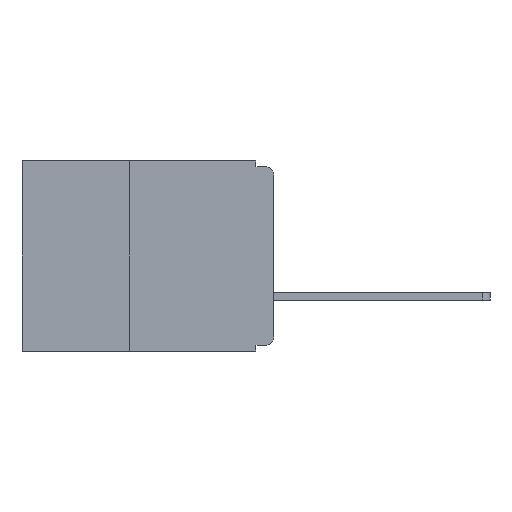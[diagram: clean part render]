
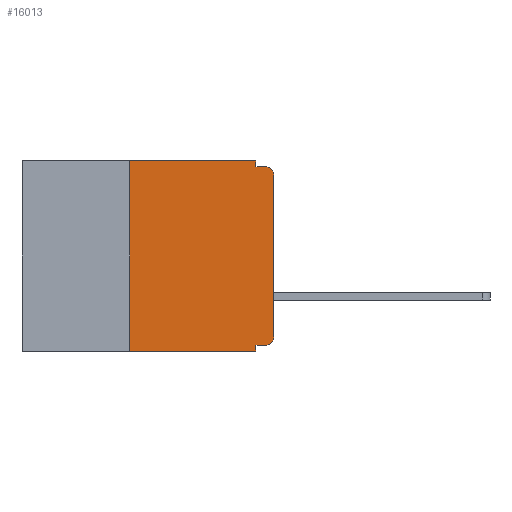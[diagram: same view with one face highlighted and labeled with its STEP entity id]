
A CAD part, left-side view. The second image highlights one B-rep face of the part: STEP entity #16013.
In plain terms, the highlighted planar face has unit normal (-1, 0, 0).
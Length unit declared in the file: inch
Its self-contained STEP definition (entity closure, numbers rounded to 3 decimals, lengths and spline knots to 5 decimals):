
#114 = ORIENTED_EDGE ( 'NONE', *, *, #16668, .T. ) ;
#137 = DIRECTION ( 'NONE',  ( 1., 0., 0. ) ) ;
#272 = CARTESIAN_POINT ( 'NONE',  ( 0., 0., -0.01 ) ) ;
#678 = VERTEX_POINT ( 'NONE', #17223 ) ;
#1757 = CARTESIAN_POINT ( 'NONE',  ( 0., 0.437, -0.33 ) ) ;
#1976 = VECTOR ( 'NONE', #2383, 39.37008 ) ;
#2167 = CARTESIAN_POINT ( 'NONE',  ( 0., 0.25, -0.33 ) ) ;
#2374 = VECTOR ( 'NONE', #10264, 39.37008 ) ;
#2383 = DIRECTION ( 'NONE',  ( 0., -1., 0. ) ) ;
#3712 = VERTEX_POINT ( 'NONE', #26113 ) ;
#4060 = CARTESIAN_POINT ( 'NONE',  ( 0., 0.437, 0. ) ) ;
#4371 = DIRECTION ( 'NONE',  ( 0., 0., -1. ) ) ;
#4772 = ORIENTED_EDGE ( 'NONE', *, *, #26075, .F. ) ;
#5046 = CARTESIAN_POINT ( 'NONE',  ( 0., 0.015, -0.32 ) ) ;
#5273 = EDGE_CURVE ( 'NONE', #24121, #24599, #18374, .T. ) ;
#5412 = CARTESIAN_POINT ( 'NONE',  ( 0., 0.015, -0.01 ) ) ;
#5504 = CARTESIAN_POINT ( 'NONE',  ( 0., 0., -0.305 ) ) ;
#5702 = ORIENTED_EDGE ( 'NONE', *, *, #24195, .T. ) ;
#5765 = ORIENTED_EDGE ( 'NONE', *, *, #13724, .F. ) ;
#5928 = EDGE_CURVE ( 'NONE', #8922, #3712, #12627, .T. ) ;
#6263 = VERTEX_POINT ( 'NONE', #5504 ) ;
#7108 = EDGE_CURVE ( 'NONE', #18911, #24121, #21765, .T. ) ;
#7191 = VERTEX_POINT ( 'NONE', #15669 ) ;
#7644 = VERTEX_POINT ( 'NONE', #23630 ) ;
#7663 = ORIENTED_EDGE ( 'NONE', *, *, #5273, .F. ) ;
#7872 = AXIS2_PLACEMENT_3D ( 'NONE', #8606, #22860, #10690 ) ;
#8042 = DIRECTION ( 'NONE',  ( 0., -1., 0. ) ) ;
#8606 = CARTESIAN_POINT ( 'NONE',  ( 0., 0.015, -0.025 ) ) ;
#8641 = CARTESIAN_POINT ( 'NONE',  ( 0., 0., -0.32 ) ) ;
#8922 = VERTEX_POINT ( 'NONE', #5046 ) ;
#8934 = LINE ( 'NONE', #25769, #25179 ) ;
#9627 = CARTESIAN_POINT ( 'NONE',  ( 0., 0.031, -0.01 ) ) ;
#9970 = CARTESIAN_POINT ( 'NONE',  ( 0., 0.015, -0.305 ) ) ;
#10036 = LINE ( 'NONE', #1757, #20617 ) ;
#10264 = DIRECTION ( 'NONE',  ( 0., 0., -1. ) ) ;
#10690 = DIRECTION ( 'NONE',  ( 0., 0., -1. ) ) ;
#10937 = CIRCLE ( 'NONE', #24810, 0.015 ) ;
#12020 = DIRECTION ( 'NONE',  ( 0., 0., -1. ) ) ;
#12032 = EDGE_CURVE ( 'NONE', #12923, #7644, #10036, .T. ) ;
#12591 = CARTESIAN_POINT ( 'NONE',  ( 0., 0.437, 0. ) ) ;
#12626 = CARTESIAN_POINT ( 'NONE',  ( 0., 0.031, 0. ) ) ;
#12627 = LINE ( 'NONE', #8641, #22792 ) ;
#12755 = LINE ( 'NONE', #16307, #2374 ) ;
#12923 = VERTEX_POINT ( 'NONE', #2167 ) ;
#13618 = DIRECTION ( 'NONE',  ( 0., 0., 1. ) ) ;
#13646 = VECTOR ( 'NONE', #22531, 39.37008 ) ;
#13724 = EDGE_CURVE ( 'NONE', #12923, #678, #8934, .T. ) ;
#14051 = ORIENTED_EDGE ( 'NONE', *, *, #18805, .T. ) ;
#14412 = AXIS2_PLACEMENT_3D ( 'NONE', #12591, #137, #14655 ) ;
#14655 = DIRECTION ( 'NONE',  ( 0., 0., -1. ) ) ;
#15669 = CARTESIAN_POINT ( 'NONE',  ( 0., 0., -0.025 ) ) ;
#16013 = ADVANCED_FACE ( 'NONE', ( #25985 ), #20676, .F. ) ;
#16049 = DIRECTION ( 'NONE',  ( 0., 0., 1. ) ) ;
#16307 = CARTESIAN_POINT ( 'NONE',  ( 0., 0.031, -0.33 ) ) ;
#16668 = EDGE_CURVE ( 'NONE', #7191, #24599, #25005, .T. ) ;
#17105 = LINE ( 'NONE', #26169, #21230 ) ;
#17223 = CARTESIAN_POINT ( 'NONE',  ( 0., 0.25, 0. ) ) ;
#18302 = EDGE_LOOP ( 'NONE', ( #5702, #114, #7663, #21236, #4772, #5765, #26265, #18310, #24473, #14051 ) ) ;
#18310 = ORIENTED_EDGE ( 'NONE', *, *, #22620, .F. ) ;
#18374 = LINE ( 'NONE', #272, #1976 ) ;
#18805 = EDGE_CURVE ( 'NONE', #8922, #6263, #10937, .T. ) ;
#18911 = VERTEX_POINT ( 'NONE', #20289 ) ;
#19040 = LINE ( 'NONE', #4060, #13646 ) ;
#20289 = CARTESIAN_POINT ( 'NONE',  ( 0., 0.031, 0. ) ) ;
#20617 = VECTOR ( 'NONE', #8042, 39.37008 ) ;
#20676 = PLANE ( 'NONE',  #14412 ) ;
#21144 = VECTOR ( 'NONE', #4371, 39.37008 ) ;
#21230 = VECTOR ( 'NONE', #16049, 39.37008 ) ;
#21236 = ORIENTED_EDGE ( 'NONE', *, *, #7108, .F. ) ;
#21765 = LINE ( 'NONE', #12626, #21144 ) ;
#22531 = DIRECTION ( 'NONE',  ( 0., -1., 0. ) ) ;
#22620 = EDGE_CURVE ( 'NONE', #3712, #7644, #12755, .T. ) ;
#22792 = VECTOR ( 'NONE', #22892, 39.37008 ) ;
#22860 = DIRECTION ( 'NONE',  ( -1., 0., 0. ) ) ;
#22892 = DIRECTION ( 'NONE',  ( 0., 1., 0. ) ) ;
#23630 = CARTESIAN_POINT ( 'NONE',  ( 0., 0.031, -0.33 ) ) ;
#24121 = VERTEX_POINT ( 'NONE', #9627 ) ;
#24189 = DIRECTION ( 'NONE',  ( -1., 0., 0. ) ) ;
#24195 = EDGE_CURVE ( 'NONE', #6263, #7191, #17105, .T. ) ;
#24473 = ORIENTED_EDGE ( 'NONE', *, *, #5928, .F. ) ;
#24599 = VERTEX_POINT ( 'NONE', #5412 ) ;
#24810 = AXIS2_PLACEMENT_3D ( 'NONE', #9970, #24189, #12020 ) ;
#25005 = CIRCLE ( 'NONE', #7872, 0.015 ) ;
#25179 = VECTOR ( 'NONE', #13618, 39.37008 ) ;
#25769 = CARTESIAN_POINT ( 'NONE',  ( 0., 0.25, -0.33 ) ) ;
#25985 = FACE_OUTER_BOUND ( 'NONE', #18302, .T. ) ;
#26075 = EDGE_CURVE ( 'NONE', #678, #18911, #19040, .T. ) ;
#26113 = CARTESIAN_POINT ( 'NONE',  ( 0., 0.031, -0.32 ) ) ;
#26169 = CARTESIAN_POINT ( 'NONE',  ( 0., 0., 0. ) ) ;
#26265 = ORIENTED_EDGE ( 'NONE', *, *, #12032, .T. ) ;
